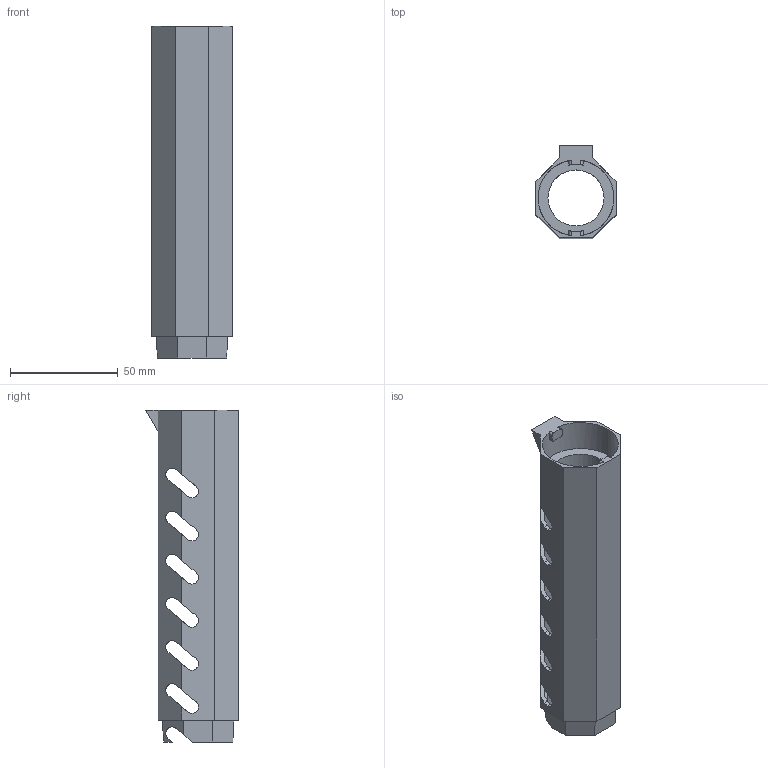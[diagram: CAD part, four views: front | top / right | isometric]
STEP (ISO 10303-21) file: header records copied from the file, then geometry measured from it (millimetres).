
FILE_DESCRIPTION (( 'STEP AP214' ), '1' );
FILE_NAME ('Handguard_Rear.step', '2019-12-18T03:07:57', ( '' ), ( '' ), 'SwSTEP 2.0', 'SolidWorks 2019', '' );
FILE_SCHEMA (( 'AUTOMOTIVE_DESIGN' ));
Length unit declared in the file: millimetre
Products named in the file (1): Handguard_Rear
Bounding box: 37.15 x 42.89 x 154 mm (x, y, z)
Volume: 37582.2 mm3; surface area: 35135.6 mm2
Topology: 2 solids, 2 shells, 154 faces, 491 edges, 316 vertices
Faces by surface type: plane 103, cylinder 51
Entity records: 5548 total; most frequent: CARTESIAN_POINT 1213, ORIENTED_EDGE 982, DIRECTION 817, EDGE_CURVE 491, VECTOR 377, LINE 377, VERTEX_POINT 316, AXIS2_PLACEMENT_3D 220
